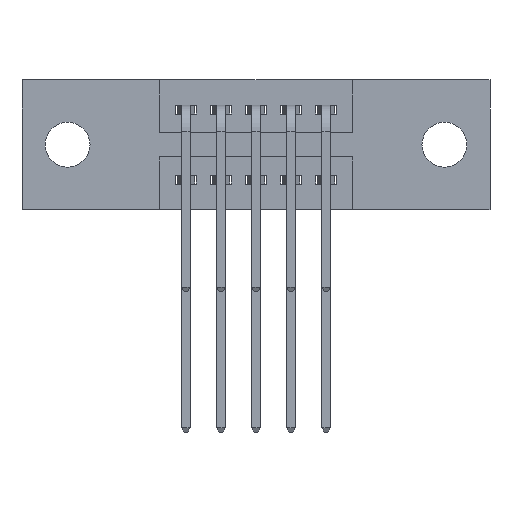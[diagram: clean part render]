
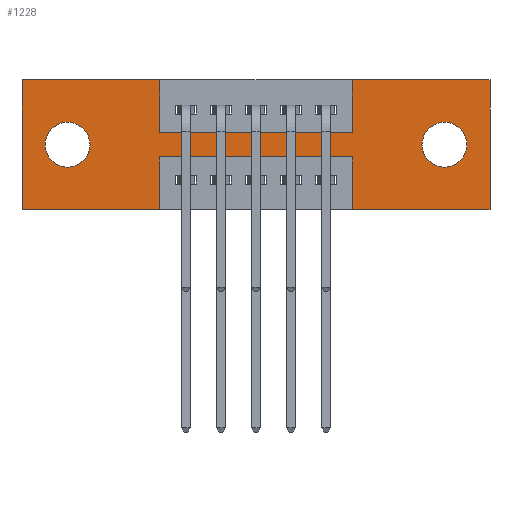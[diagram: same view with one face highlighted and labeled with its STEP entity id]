
A CAD part, front view. The second image highlights one B-rep face of the part: STEP entity #1228.
In plain terms, the highlighted planar face has unit normal (0, -1, 0).
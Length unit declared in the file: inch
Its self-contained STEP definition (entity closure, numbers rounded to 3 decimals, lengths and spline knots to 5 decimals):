
#65 = CARTESIAN_POINT ( 'NONE',  ( 0., 0., 0. ) ) ;
#183 = CARTESIAN_POINT ( 'NONE',  ( 0., 0., -0.37 ) ) ;
#217 = VERTEX_POINT ( 'NONE', #1266 ) ;
#224 = VECTOR ( 'NONE', #1849, 39.37008 ) ;
#313 = EDGE_CURVE ( 'NONE', #217, #3060, #10016, .T. ) ;
#395 = VERTEX_POINT ( 'NONE', #907 ) ;
#438 = LINE ( 'NONE', #966, #2103 ) ;
#484 = ORIENTED_EDGE ( 'NONE', *, *, #4661, .F. ) ;
#505 = LINE ( 'NONE', #9961, #2287 ) ;
#540 = DIRECTION ( 'NONE',  ( 0., 1., 0. ) ) ;
#559 = CIRCLE ( 'NONE', #6744, 0.064 ) ;
#842 = DIRECTION ( 'NONE',  ( 0., 0., 1. ) ) ;
#853 = EDGE_CURVE ( 'NONE', #5872, #2847, #438, .T. ) ;
#884 = CARTESIAN_POINT ( 'NONE',  ( 1.205, 0., -0.185 ) ) ;
#907 = CARTESIAN_POINT ( 'NONE',  ( 0.3925, 0., 0. ) ) ;
#966 = CARTESIAN_POINT ( 'NONE',  ( 0.9425, 0., 0. ) ) ;
#1008 = VECTOR ( 'NONE', #4501, 39.37008 ) ;
#1116 = CARTESIAN_POINT ( 'NONE',  ( 0.3925, 0., -0.37 ) ) ;
#1159 = ORIENTED_EDGE ( 'NONE', *, *, #3882, .F. ) ;
#1205 = CARTESIAN_POINT ( 'NONE',  ( 0.3925, 0., -0.15 ) ) ;
#1228 = ADVANCED_FACE ( 'NONE', ( #3775, #10378, #2734 ), #3985, .T. ) ;
#1266 = CARTESIAN_POINT ( 'NONE',  ( 1.205, 0., -0.249 ) ) ;
#1348 = CARTESIAN_POINT ( 'NONE',  ( 0.13, 0., -0.249 ) ) ;
#1363 = ORIENTED_EDGE ( 'NONE', *, *, #5760, .F. ) ;
#1468 = ORIENTED_EDGE ( 'NONE', *, *, #3079, .T. ) ;
#1598 = CARTESIAN_POINT ( 'NONE',  ( 0.13, 0., -0.121 ) ) ;
#1608 = DIRECTION ( 'NONE',  ( 1., 0., 0. ) ) ;
#1702 = CARTESIAN_POINT ( 'NONE',  ( 0.3925, 0., -0.22 ) ) ;
#1745 = VERTEX_POINT ( 'NONE', #5774 ) ;
#1775 = DIRECTION ( 'NONE',  ( 0., 0., 1. ) ) ;
#1837 = EDGE_CURVE ( 'NONE', #1920, #6224, #7441, .T. ) ;
#1849 = DIRECTION ( 'NONE',  ( 0., 0., 1. ) ) ;
#1920 = VERTEX_POINT ( 'NONE', #7690 ) ;
#1942 = VERTEX_POINT ( 'NONE', #5313 ) ;
#2036 = DIRECTION ( 'NONE',  ( 0., 1., 0. ) ) ;
#2052 = CARTESIAN_POINT ( 'NONE',  ( 1.335, 0., 0. ) ) ;
#2103 = VECTOR ( 'NONE', #1775, 39.37008 ) ;
#2130 = EDGE_LOOP ( 'NONE', ( #9439, #6948 ) ) ;
#2287 = VECTOR ( 'NONE', #5736, 39.37008 ) ;
#2317 = CARTESIAN_POINT ( 'NONE',  ( 0., 0., 0. ) ) ;
#2537 = EDGE_CURVE ( 'NONE', #6224, #7848, #9701, .T. ) ;
#2555 = ORIENTED_EDGE ( 'NONE', *, *, #1837, .F. ) ;
#2605 = VERTEX_POINT ( 'NONE', #9534 ) ;
#2686 = ORIENTED_EDGE ( 'NONE', *, *, #5612, .F. ) ;
#2734 = FACE_OUTER_BOUND ( 'NONE', #8938, .T. ) ;
#2797 = CARTESIAN_POINT ( 'NONE',  ( 0.9425, 0., -0.15 ) ) ;
#2847 = VERTEX_POINT ( 'NONE', #9043 ) ;
#2904 = LINE ( 'NONE', #2052, #1008 ) ;
#2911 = DIRECTION ( 'NONE',  ( 0., 0., 1. ) ) ;
#3060 = VERTEX_POINT ( 'NONE', #4484 ) ;
#3079 = EDGE_CURVE ( 'NONE', #4318, #8234, #8042, .T. ) ;
#3187 = CARTESIAN_POINT ( 'NONE',  ( 0., 0., -0.37 ) ) ;
#3775 = FACE_BOUND ( 'NONE', #2130, .T. ) ;
#3882 = EDGE_CURVE ( 'NONE', #2847, #2605, #7898, .T. ) ;
#3942 = AXIS2_PLACEMENT_3D ( 'NONE', #10297, #540, #9440 ) ;
#3966 = VERTEX_POINT ( 'NONE', #9898 ) ;
#3985 = PLANE ( 'NONE',  #9182 ) ;
#4318 = VERTEX_POINT ( 'NONE', #1598 ) ;
#4484 = CARTESIAN_POINT ( 'NONE',  ( 1.205, 0., -0.121 ) ) ;
#4501 = DIRECTION ( 'NONE',  ( 0., 0., -1. ) ) ;
#4511 = EDGE_CURVE ( 'NONE', #1745, #3966, #5090, .T. ) ;
#4515 = VERTEX_POINT ( 'NONE', #6733 ) ;
#4562 = ORIENTED_EDGE ( 'NONE', *, *, #9235, .F. ) ;
#4582 = EDGE_CURVE ( 'NONE', #2605, #1942, #2904, .T. ) ;
#4661 = EDGE_CURVE ( 'NONE', #4515, #5872, #4831, .T. ) ;
#4831 = LINE ( 'NONE', #1205, #5987 ) ;
#5052 = EDGE_LOOP ( 'NONE', ( #1468, #7218 ) ) ;
#5090 = LINE ( 'NONE', #6771, #224 ) ;
#5136 = CARTESIAN_POINT ( 'NONE',  ( 0.9425, 0., -0.37 ) ) ;
#5154 = DIRECTION ( 'NONE',  ( -1., 0., 0. ) ) ;
#5177 = CARTESIAN_POINT ( 'NONE',  ( 0., 0., -0.37 ) ) ;
#5237 = VECTOR ( 'NONE', #1608, 39.37008 ) ;
#5313 = CARTESIAN_POINT ( 'NONE',  ( 1.335, 0., -0.37 ) ) ;
#5484 = VECTOR ( 'NONE', #5861, 39.37008 ) ;
#5509 = VECTOR ( 'NONE', #8668, 39.37008 ) ;
#5612 = EDGE_CURVE ( 'NONE', #3966, #395, #5743, .T. ) ;
#5688 = AXIS2_PLACEMENT_3D ( 'NONE', #10531, #10566, #842 ) ;
#5736 = DIRECTION ( 'NONE',  ( 0., 0., -1. ) ) ;
#5743 = LINE ( 'NONE', #2317, #5237 ) ;
#5760 = EDGE_CURVE ( 'NONE', #395, #4515, #505, .T. ) ;
#5774 = CARTESIAN_POINT ( 'NONE',  ( 0., 0., -0.37 ) ) ;
#5861 = DIRECTION ( 'NONE',  ( 1., 0., 0. ) ) ;
#5872 = VERTEX_POINT ( 'NONE', #2797 ) ;
#5987 = VECTOR ( 'NONE', #7643, 39.37008 ) ;
#6006 = AXIS2_PLACEMENT_3D ( 'NONE', #9359, #2036, #2911 ) ;
#6080 = VECTOR ( 'NONE', #7625, 39.37008 ) ;
#6224 = VERTEX_POINT ( 'NONE', #8881 ) ;
#6262 = EDGE_CURVE ( 'NONE', #8234, #4318, #9410, .T. ) ;
#6343 = DIRECTION ( 'NONE',  ( 0., -1., 0. ) ) ;
#6389 = EDGE_CURVE ( 'NONE', #7848, #6491, #8772, .T. ) ;
#6393 = VECTOR ( 'NONE', #8382, 39.37008 ) ;
#6410 = ORIENTED_EDGE ( 'NONE', *, *, #2537, .F. ) ;
#6436 = VECTOR ( 'NONE', #8555, 39.37008 ) ;
#6491 = VERTEX_POINT ( 'NONE', #1116 ) ;
#6597 = DIRECTION ( 'NONE',  ( 0., 0., -1. ) ) ;
#6733 = CARTESIAN_POINT ( 'NONE',  ( 0.3925, 0., -0.15 ) ) ;
#6744 = AXIS2_PLACEMENT_3D ( 'NONE', #884, #9061, #6597 ) ;
#6771 = CARTESIAN_POINT ( 'NONE',  ( 0., 0., 0. ) ) ;
#6948 = ORIENTED_EDGE ( 'NONE', *, *, #313, .T. ) ;
#7051 = ORIENTED_EDGE ( 'NONE', *, *, #853, .F. ) ;
#7218 = ORIENTED_EDGE ( 'NONE', *, *, #6262, .T. ) ;
#7219 = LINE ( 'NONE', #5177, #6080 ) ;
#7441 = LINE ( 'NONE', #5136, #6436 ) ;
#7619 = ORIENTED_EDGE ( 'NONE', *, *, #4582, .F. ) ;
#7625 = DIRECTION ( 'NONE',  ( -1., 0., 0. ) ) ;
#7627 = CARTESIAN_POINT ( 'NONE',  ( 0.3925, 0., -0.37 ) ) ;
#7642 = ORIENTED_EDGE ( 'NONE', *, *, #4511, .F. ) ;
#7643 = DIRECTION ( 'NONE',  ( 1., 0., 0. ) ) ;
#7690 = CARTESIAN_POINT ( 'NONE',  ( 0.9425, 0., -0.37 ) ) ;
#7848 = VERTEX_POINT ( 'NONE', #1702 ) ;
#7898 = LINE ( 'NONE', #65, #5484 ) ;
#8042 = CIRCLE ( 'NONE', #6006, 0.064 ) ;
#8234 = VERTEX_POINT ( 'NONE', #1348 ) ;
#8286 = ORIENTED_EDGE ( 'NONE', *, *, #6389, .F. ) ;
#8382 = DIRECTION ( 'NONE',  ( 0., 0., -1. ) ) ;
#8555 = DIRECTION ( 'NONE',  ( 0., 0., 1. ) ) ;
#8666 = EDGE_CURVE ( 'NONE', #6491, #1745, #10014, .T. ) ;
#8668 = DIRECTION ( 'NONE',  ( -1., 0., 0. ) ) ;
#8772 = LINE ( 'NONE', #7627, #6393 ) ;
#8881 = CARTESIAN_POINT ( 'NONE',  ( 0.9425, 0., -0.22 ) ) ;
#8938 = EDGE_LOOP ( 'NONE', ( #8286, #6410, #2555, #4562, #7619, #1159, #7051, #484, #1363, #2686, #7642, #10160 ) ) ;
#9043 = CARTESIAN_POINT ( 'NONE',  ( 0.9425, 0., 0. ) ) ;
#9061 = DIRECTION ( 'NONE',  ( 0., 1., 0. ) ) ;
#9182 = AXIS2_PLACEMENT_3D ( 'NONE', #3187, #6343, #10385 ) ;
#9235 = EDGE_CURVE ( 'NONE', #1942, #1920, #7219, .T. ) ;
#9359 = CARTESIAN_POINT ( 'NONE',  ( 0.13, 0., -0.185 ) ) ;
#9400 = CARTESIAN_POINT ( 'NONE',  ( 0.3925, 0., -0.22 ) ) ;
#9410 = CIRCLE ( 'NONE', #5688, 0.064 ) ;
#9439 = ORIENTED_EDGE ( 'NONE', *, *, #9768, .T. ) ;
#9440 = DIRECTION ( 'NONE',  ( 0., 0., -1. ) ) ;
#9534 = CARTESIAN_POINT ( 'NONE',  ( 1.335, 0., 0. ) ) ;
#9701 = LINE ( 'NONE', #9400, #5509 ) ;
#9749 = VECTOR ( 'NONE', #5154, 39.37008 ) ;
#9768 = EDGE_CURVE ( 'NONE', #3060, #217, #559, .T. ) ;
#9898 = CARTESIAN_POINT ( 'NONE',  ( 0., 0., 0. ) ) ;
#9961 = CARTESIAN_POINT ( 'NONE',  ( 0.3925, 0., 0. ) ) ;
#10014 = LINE ( 'NONE', #183, #9749 ) ;
#10016 = CIRCLE ( 'NONE', #3942, 0.064 ) ;
#10160 = ORIENTED_EDGE ( 'NONE', *, *, #8666, .F. ) ;
#10297 = CARTESIAN_POINT ( 'NONE',  ( 1.205, 0., -0.185 ) ) ;
#10378 = FACE_BOUND ( 'NONE', #5052, .T. ) ;
#10385 = DIRECTION ( 'NONE',  ( 0., 0., -1. ) ) ;
#10531 = CARTESIAN_POINT ( 'NONE',  ( 0.13, 0., -0.185 ) ) ;
#10566 = DIRECTION ( 'NONE',  ( 0., 1., 0. ) ) ;
